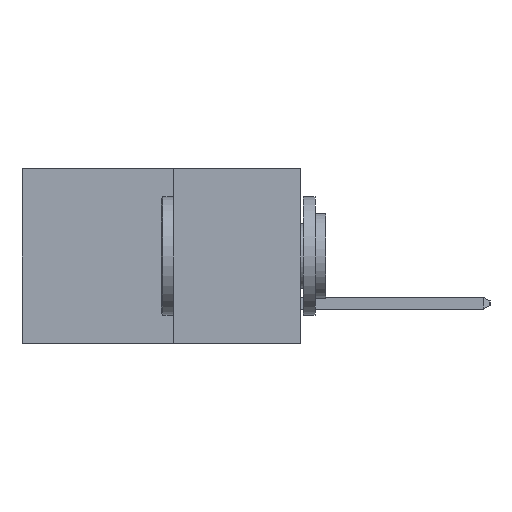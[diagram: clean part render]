
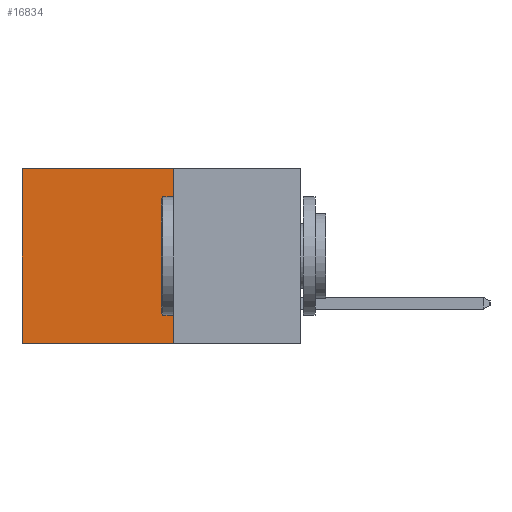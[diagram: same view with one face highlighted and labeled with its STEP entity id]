
A CAD part, left-side view. The second image highlights one B-rep face of the part: STEP entity #16834.
In plain terms, the highlighted planar face has unit normal (-1, 0, 0).
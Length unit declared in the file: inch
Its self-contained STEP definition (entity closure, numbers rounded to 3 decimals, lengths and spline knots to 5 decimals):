
#124 = EDGE_CURVE ( 'NONE', #3407, #7727, #7840, .T. ) ;
#806 = AXIS2_PLACEMENT_3D ( 'NONE', #13608, #5057, #15009 ) ;
#2027 = CARTESIAN_POINT ( 'NONE',  ( 0.277, 0.59, -0.37 ) ) ;
#3211 = DIRECTION ( 'NONE',  ( 0., 1., 0. ) ) ;
#3407 = VERTEX_POINT ( 'NONE', #7694 ) ;
#4862 = ORIENTED_EDGE ( 'NONE', *, *, #11075, .F. ) ;
#5057 = DIRECTION ( 'NONE',  ( 1., 0., 0. ) ) ;
#5472 = CARTESIAN_POINT ( 'NONE',  ( 0.277, 0.27, -0.37 ) ) ;
#6725 = EDGE_CURVE ( 'NONE', #11712, #8417, #8468, .T. ) ;
#6843 = ORIENTED_EDGE ( 'NONE', *, *, #6725, .T. ) ;
#6875 = DIRECTION ( 'NONE',  ( 0., 1., 0. ) ) ;
#7694 = CARTESIAN_POINT ( 'NONE',  ( 0.277, 0.27, 0. ) ) ;
#7727 = VERTEX_POINT ( 'NONE', #10679 ) ;
#7840 = LINE ( 'NONE', #12373, #12098 ) ;
#8417 = VERTEX_POINT ( 'NONE', #2027 ) ;
#8468 = LINE ( 'NONE', #11161, #16013 ) ;
#8558 = FACE_OUTER_BOUND ( 'NONE', #10836, .T. ) ;
#8733 = VECTOR ( 'NONE', #6875, 39.37008 ) ;
#9189 = LINE ( 'NONE', #5472, #8733 ) ;
#9475 = EDGE_CURVE ( 'NONE', #3407, #11712, #13917, .T. ) ;
#10110 = VECTOR ( 'NONE', #3211, 39.37008 ) ;
#10679 = CARTESIAN_POINT ( 'NONE',  ( 0.277, 0.27, -0.37 ) ) ;
#10706 = PLANE ( 'NONE',  #806 ) ;
#10836 = EDGE_LOOP ( 'NONE', ( #6843, #4862, #17200, #11362 ) ) ;
#11075 = EDGE_CURVE ( 'NONE', #7727, #8417, #9189, .T. ) ;
#11161 = CARTESIAN_POINT ( 'NONE',  ( 0.277, 0.59, -0.37 ) ) ;
#11165 = DIRECTION ( 'NONE',  ( 0., 0., -1. ) ) ;
#11362 = ORIENTED_EDGE ( 'NONE', *, *, #9475, .T. ) ;
#11712 = VERTEX_POINT ( 'NONE', #16784 ) ;
#12098 = VECTOR ( 'NONE', #12218, 39.37008 ) ;
#12218 = DIRECTION ( 'NONE',  ( 0., 0., -1. ) ) ;
#12373 = CARTESIAN_POINT ( 'NONE',  ( 0.277, 0.27, -0.37 ) ) ;
#13608 = CARTESIAN_POINT ( 'NONE',  ( 0.277, 0.27, -0.37 ) ) ;
#13917 = LINE ( 'NONE', #17431, #10110 ) ;
#15009 = DIRECTION ( 'NONE',  ( 0., 0., -1. ) ) ;
#16013 = VECTOR ( 'NONE', #11165, 39.37008 ) ;
#16784 = CARTESIAN_POINT ( 'NONE',  ( 0.277, 0.59, 0. ) ) ;
#16834 = ADVANCED_FACE ( 'NONE', ( #8558 ), #10706, .F. ) ;
#17200 = ORIENTED_EDGE ( 'NONE', *, *, #124, .F. ) ;
#17431 = CARTESIAN_POINT ( 'NONE',  ( 0.277, 0.27, 0. ) ) ;
